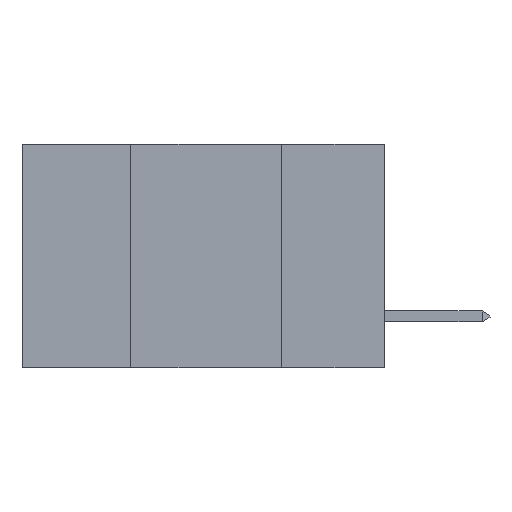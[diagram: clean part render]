
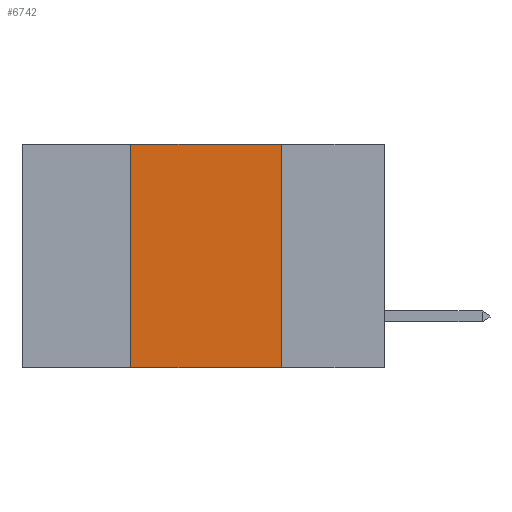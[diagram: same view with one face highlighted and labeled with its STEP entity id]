
A CAD part, left-side view. The second image highlights one B-rep face of the part: STEP entity #6742.
In plain terms, the highlighted planar face has unit normal (-1, 0, 0).
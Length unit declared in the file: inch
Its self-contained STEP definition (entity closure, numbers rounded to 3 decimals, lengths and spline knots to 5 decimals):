
#54 = FACE_OUTER_BOUND ( 'NONE', #11995, .T. ) ;
#194 = DIRECTION ( 'NONE',  ( 0., 0., -1. ) ) ;
#466 = DIRECTION ( 'NONE',  ( 0., 0., 1. ) ) ;
#717 = EDGE_CURVE ( 'NONE', #19172, #6149, #5502, .T. ) ;
#948 = LINE ( 'NONE', #6422, #7528 ) ;
#1970 = ORIENTED_EDGE ( 'NONE', *, *, #3132, .F. ) ;
#2220 = EDGE_CURVE ( 'NONE', #19172, #13575, #12365, .T. ) ;
#2550 = VECTOR ( 'NONE', #10927, 39.37008 ) ;
#2870 = ORIENTED_EDGE ( 'NONE', *, *, #14204, .F. ) ;
#3132 = EDGE_CURVE ( 'NONE', #7366, #6149, #948, .T. ) ;
#3719 = ORIENTED_EDGE ( 'NONE', *, *, #717, .T. ) ;
#4077 = AXIS2_PLACEMENT_3D ( 'NONE', #16843, #18533, #194 ) ;
#5502 = LINE ( 'NONE', #13342, #16650 ) ;
#6149 = VERTEX_POINT ( 'NONE', #11309 ) ;
#6422 = CARTESIAN_POINT ( 'NONE',  ( 0., 0.17, 0. ) ) ;
#6742 = ADVANCED_FACE ( 'NONE', ( #54 ), #20451, .F. ) ;
#7160 = CARTESIAN_POINT ( 'NONE',  ( 0., 0.42, 0. ) ) ;
#7217 = CARTESIAN_POINT ( 'NONE',  ( 0., 0.42, -0.37 ) ) ;
#7366 = VERTEX_POINT ( 'NONE', #16929 ) ;
#7528 = VECTOR ( 'NONE', #14766, 39.37008 ) ;
#7570 = VECTOR ( 'NONE', #466, 39.37008 ) ;
#10927 = DIRECTION ( 'NONE',  ( 0., -1., 0. ) ) ;
#11309 = CARTESIAN_POINT ( 'NONE',  ( 0., 0.17, -0.37 ) ) ;
#11995 = EDGE_LOOP ( 'NONE', ( #1970, #2870, #15922, #3719 ) ) ;
#12365 = LINE ( 'NONE', #7160, #7570 ) ;
#12575 = CARTESIAN_POINT ( 'NONE',  ( 0., 0.42, 0. ) ) ;
#13342 = CARTESIAN_POINT ( 'NONE',  ( 0., 0.6, -0.37 ) ) ;
#13575 = VERTEX_POINT ( 'NONE', #12575 ) ;
#14204 = EDGE_CURVE ( 'NONE', #13575, #7366, #17365, .T. ) ;
#14766 = DIRECTION ( 'NONE',  ( 0., 0., -1. ) ) ;
#15212 = DIRECTION ( 'NONE',  ( 0., -1., 0. ) ) ;
#15922 = ORIENTED_EDGE ( 'NONE', *, *, #2220, .F. ) ;
#16650 = VECTOR ( 'NONE', #15212, 39.37008 ) ;
#16843 = CARTESIAN_POINT ( 'NONE',  ( 0., 0.6, 0. ) ) ;
#16929 = CARTESIAN_POINT ( 'NONE',  ( 0., 0.17, 0. ) ) ;
#17365 = LINE ( 'NONE', #17610, #2550 ) ;
#17610 = CARTESIAN_POINT ( 'NONE',  ( 0., 0.6, 0. ) ) ;
#18533 = DIRECTION ( 'NONE',  ( 1., 0., 0. ) ) ;
#19172 = VERTEX_POINT ( 'NONE', #7217 ) ;
#20451 = PLANE ( 'NONE',  #4077 ) ;
